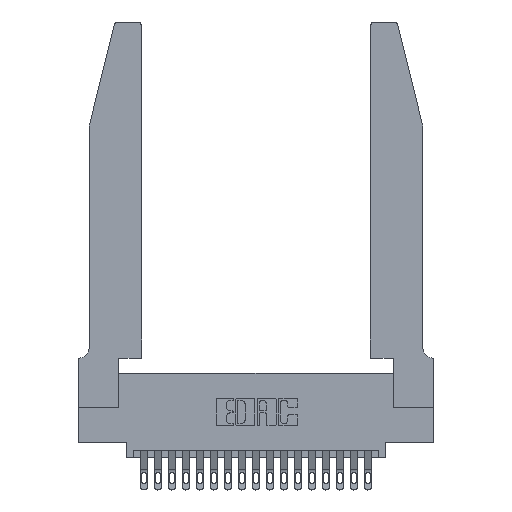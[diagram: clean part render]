
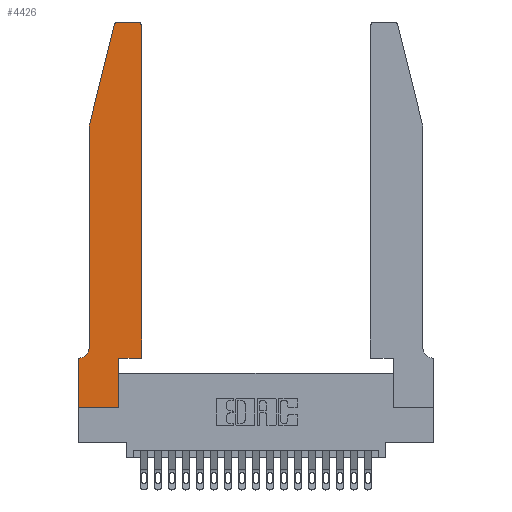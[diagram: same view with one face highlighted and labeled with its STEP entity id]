
A CAD part, top view. The second image highlights one B-rep face of the part: STEP entity #4426.
In plain terms, the highlighted planar face has unit normal (0, 0, 1).
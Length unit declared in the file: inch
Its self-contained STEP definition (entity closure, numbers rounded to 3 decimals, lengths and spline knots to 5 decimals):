
#62 = AXIS2_PLACEMENT_3D ( 'NONE', #4667, #11159, #1249 ) ;
#156 = VECTOR ( 'NONE', #19427, 39.37008 ) ;
#357 = DIRECTION ( 'NONE',  ( 1., 0., 0. ) ) ;
#982 = DIRECTION ( 'NONE',  ( 0., 0., 1. ) ) ;
#1012 = VECTOR ( 'NONE', #7304, 39.37008 ) ;
#1106 = EDGE_CURVE ( 'NONE', #1306, #11207, #7255, .T. ) ;
#1249 = DIRECTION ( 'NONE',  ( 1., 0., 0. ) ) ;
#1306 = VERTEX_POINT ( 'NONE', #12819 ) ;
#1347 = CARTESIAN_POINT ( 'NONE',  ( 0., 0., 0.37 ) ) ;
#1787 = VERTEX_POINT ( 'NONE', #4252 ) ;
#2055 = VECTOR ( 'NONE', #8303, 39.37008 ) ;
#2075 = LINE ( 'NONE', #10593, #1012 ) ;
#2193 = ORIENTED_EDGE ( 'NONE', *, *, #2387, .T. ) ;
#2387 = EDGE_CURVE ( 'NONE', #19602, #8305, #8506, .T. ) ;
#2690 = CARTESIAN_POINT ( 'NONE',  ( 0., 0.35, 0.37 ) ) ;
#2820 = VERTEX_POINT ( 'NONE', #10109 ) ;
#3007 = CIRCLE ( 'NONE', #16956, 0.07 ) ;
#3047 = CARTESIAN_POINT ( 'NONE',  ( 0.4505, 0.35, 0.37 ) ) ;
#3056 = ORIENTED_EDGE ( 'NONE', *, *, #16171, .T. ) ;
#3090 = CARTESIAN_POINT ( 'NONE',  ( 0.0055, 0.42, 0.37 ) ) ;
#3261 = DIRECTION ( 'NONE',  ( 0., -1., 0. ) ) ;
#3402 = EDGE_CURVE ( 'NONE', #2820, #13608, #3007, .T. ) ;
#3704 = CARTESIAN_POINT ( 'NONE',  ( 0.0055, 0.35, 0.37 ) ) ;
#3764 = FACE_OUTER_BOUND ( 'NONE', #9107, .T. ) ;
#4035 = CARTESIAN_POINT ( 'NONE',  ( 0.0755, 2., 0.37 ) ) ;
#4237 = ORIENTED_EDGE ( 'NONE', *, *, #10143, .T. ) ;
#4252 = CARTESIAN_POINT ( 'NONE',  ( 0.4505, 2.72, 0.37 ) ) ;
#4426 = ADVANCED_FACE ( 'NONE', ( #3764 ), #6047, .T. ) ;
#4667 = CARTESIAN_POINT ( 'NONE',  ( 0.284, 2.72, 0.37 ) ) ;
#4740 = DIRECTION ( 'NONE',  ( 0., 0., -1. ) ) ;
#4892 = VERTEX_POINT ( 'NONE', #18191 ) ;
#5125 = VECTOR ( 'NONE', #11774, 39.37008 ) ;
#5620 = ORIENTED_EDGE ( 'NONE', *, *, #3402, .T. ) ;
#6047 = PLANE ( 'NONE',  #12398 ) ;
#6053 = ORIENTED_EDGE ( 'NONE', *, *, #16312, .T. ) ;
#6155 = LINE ( 'NONE', #17951, #15641 ) ;
#6299 = ORIENTED_EDGE ( 'NONE', *, *, #13455, .T. ) ;
#6414 = EDGE_CURVE ( 'NONE', #13608, #14719, #2075, .T. ) ;
#6519 = CIRCLE ( 'NONE', #6612, 0.03 ) ;
#6612 = AXIS2_PLACEMENT_3D ( 'NONE', #17534, #10646, #357 ) ;
#6863 = EDGE_CURVE ( 'NONE', #9338, #19602, #16882, .T. ) ;
#7255 = LINE ( 'NONE', #3047, #5125 ) ;
#7304 = DIRECTION ( 'NONE',  ( -1., 0., 0. ) ) ;
#7547 = CARTESIAN_POINT ( 'NONE',  ( 0.284, 2.75, 0.37 ) ) ;
#7838 = DIRECTION ( 'NONE',  ( 0., 1., 0. ) ) ;
#8129 = VECTOR ( 'NONE', #20626, 39.37008 ) ;
#8276 = ORIENTED_EDGE ( 'NONE', *, *, #6414, .T. ) ;
#8303 = DIRECTION ( 'NONE',  ( -1., 0., 0. ) ) ;
#8305 = VERTEX_POINT ( 'NONE', #17612 ) ;
#8497 = DIRECTION ( 'NONE',  ( 1., 0., 0. ) ) ;
#8506 = CIRCLE ( 'NONE', #62, 0.03 ) ;
#8589 = CARTESIAN_POINT ( 'NONE',  ( 0.4505, 0.35, 0.37 ) ) ;
#9107 = EDGE_LOOP ( 'NONE', ( #9231, #2193, #6053, #17304, #5620, #8276, #6299, #9288, #4237, #18168, #3056, #10073 ) ) ;
#9231 = ORIENTED_EDGE ( 'NONE', *, *, #6863, .T. ) ;
#9288 = ORIENTED_EDGE ( 'NONE', *, *, #17548, .T. ) ;
#9338 = VERTEX_POINT ( 'NONE', #18407 ) ;
#9712 = LINE ( 'NONE', #10682, #8129 ) ;
#10073 = ORIENTED_EDGE ( 'NONE', *, *, #13638, .T. ) ;
#10109 = CARTESIAN_POINT ( 'NONE',  ( 0.0755, 0.42, 0.37 ) ) ;
#10143 = EDGE_CURVE ( 'NONE', #18324, #1306, #6155, .T. ) ;
#10448 = VECTOR ( 'NONE', #3261, 39.37008 ) ;
#10593 = CARTESIAN_POINT ( 'NONE',  ( 0.0755, 0.35, 0.37 ) ) ;
#10646 = DIRECTION ( 'NONE',  ( 0., 0., 1. ) ) ;
#10682 = CARTESIAN_POINT ( 'NONE',  ( 0.4505, 0.35, 0.37 ) ) ;
#11159 = DIRECTION ( 'NONE',  ( 0., 0., 1. ) ) ;
#11207 = VERTEX_POINT ( 'NONE', #8589 ) ;
#11761 = VECTOR ( 'NONE', #8497, 39.37008 ) ;
#11774 = DIRECTION ( 'NONE',  ( 1., 0., 0. ) ) ;
#11955 = CARTESIAN_POINT ( 'NONE',  ( 0., 0., 0.37 ) ) ;
#12398 = AXIS2_PLACEMENT_3D ( 'NONE', #12896, #982, #17873 ) ;
#12429 = CARTESIAN_POINT ( 'NONE',  ( 0.2865, 0., 0.37 ) ) ;
#12819 = CARTESIAN_POINT ( 'NONE',  ( 0.2865, 0.35, 0.37 ) ) ;
#12896 = CARTESIAN_POINT ( 'NONE',  ( 0., 0.35, 0.37 ) ) ;
#13247 = CARTESIAN_POINT ( 'NONE',  ( 0.2605, 2.75, 0.37 ) ) ;
#13455 = EDGE_CURVE ( 'NONE', #14719, #4892, #20818, .T. ) ;
#13608 = VERTEX_POINT ( 'NONE', #3704 ) ;
#13638 = EDGE_CURVE ( 'NONE', #1787, #9338, #6519, .T. ) ;
#13841 = CARTESIAN_POINT ( 'NONE',  ( 0.0755, 2., 0.37 ) ) ;
#13998 = VECTOR ( 'NONE', #19210, 39.37008 ) ;
#14719 = VERTEX_POINT ( 'NONE', #2690 ) ;
#15641 = VECTOR ( 'NONE', #7838, 39.37008 ) ;
#15965 = VERTEX_POINT ( 'NONE', #20036 ) ;
#16171 = EDGE_CURVE ( 'NONE', #11207, #1787, #9712, .T. ) ;
#16312 = EDGE_CURVE ( 'NONE', #8305, #15965, #21905, .T. ) ;
#16882 = LINE ( 'NONE', #13247, #2055 ) ;
#16956 = AXIS2_PLACEMENT_3D ( 'NONE', #3090, #4740, #18271 ) ;
#17304 = ORIENTED_EDGE ( 'NONE', *, *, #20805, .T. ) ;
#17534 = CARTESIAN_POINT ( 'NONE',  ( 0.4205, 2.72, 0.37 ) ) ;
#17548 = EDGE_CURVE ( 'NONE', #4892, #18324, #20264, .T. ) ;
#17612 = CARTESIAN_POINT ( 'NONE',  ( 0.25487, 2.72718, 0.37 ) ) ;
#17873 = DIRECTION ( 'NONE',  ( 1., 0., 0. ) ) ;
#17951 = CARTESIAN_POINT ( 'NONE',  ( 0.2865, 0.35, 0.37 ) ) ;
#18005 = LINE ( 'NONE', #13841, #13998 ) ;
#18168 = ORIENTED_EDGE ( 'NONE', *, *, #1106, .T. ) ;
#18191 = CARTESIAN_POINT ( 'NONE',  ( 0., 0., 0.37 ) ) ;
#18271 = DIRECTION ( 'NONE',  ( -1., 0., 0. ) ) ;
#18324 = VERTEX_POINT ( 'NONE', #12429 ) ;
#18407 = CARTESIAN_POINT ( 'NONE',  ( 0.4205, 2.75, 0.37 ) ) ;
#19210 = DIRECTION ( 'NONE',  ( 0., -1., 0. ) ) ;
#19427 = DIRECTION ( 'NONE',  ( -0.239, -0.971, 0. ) ) ;
#19602 = VERTEX_POINT ( 'NONE', #7547 ) ;
#20036 = CARTESIAN_POINT ( 'NONE',  ( 0.0755, 2., 0.37 ) ) ;
#20264 = LINE ( 'NONE', #11955, #11761 ) ;
#20626 = DIRECTION ( 'NONE',  ( 0., 1., 0. ) ) ;
#20805 = EDGE_CURVE ( 'NONE', #15965, #2820, #18005, .T. ) ;
#20818 = LINE ( 'NONE', #1347, #10448 ) ;
#21905 = LINE ( 'NONE', #4035, #156 ) ;
